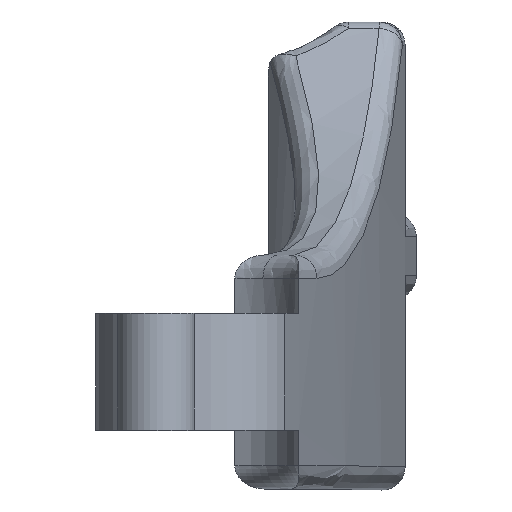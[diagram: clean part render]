
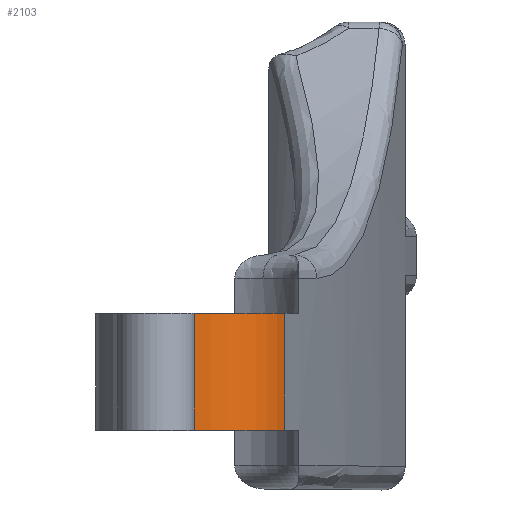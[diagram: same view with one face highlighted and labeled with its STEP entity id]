
A CAD part, top view. The second image highlights one B-rep face of the part: STEP entity #2103.
In plain terms, the highlighted cylindrical face has radius 12.6 mm (diameter 25.2 mm), a partial arc.
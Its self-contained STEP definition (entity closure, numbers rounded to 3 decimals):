
#48 = LINE ( 'NONE', #2157, #1083 ) ;
#54 = EDGE_LOOP ( 'NONE', ( #624, #430, #1079, #2313 ) ) ;
#61 = DIRECTION ( 'NONE',  ( 0., -1., 0. ) ) ;
#77 = DIRECTION ( 'NONE',  ( 0., 0., -1. ) ) ;
#184 = CARTESIAN_POINT ( 'NONE',  ( 0., 7.5, 110. ) ) ;
#252 = VERTEX_POINT ( 'NONE', #868 ) ;
#430 = ORIENTED_EDGE ( 'NONE', *, *, #2068, .T. ) ;
#481 = VERTEX_POINT ( 'NONE', #1852 ) ;
#607 = EDGE_CURVE ( 'NONE', #2057, #481, #1651, .T. ) ;
#624 = ORIENTED_EDGE ( 'NONE', *, *, #607, .T. ) ;
#700 = CARTESIAN_POINT ( 'NONE',  ( 0., 22.5, 110. ) ) ;
#797 = EDGE_CURVE ( 'NONE', #1496, #252, #1584, .T. ) ;
#868 = CARTESIAN_POINT ( 'NONE',  ( 0.037, 7.5, 122.6 ) ) ;
#874 = AXIS2_PLACEMENT_3D ( 'NONE', #700, #1478, #2463 ) ;
#1079 = ORIENTED_EDGE ( 'NONE', *, *, #797, .F. ) ;
#1083 = VECTOR ( 'NONE', #1208, 1000. ) ;
#1156 = CARTESIAN_POINT ( 'NONE',  ( 11.668, 7.5, 114.755 ) ) ;
#1175 = EDGE_CURVE ( 'NONE', #2057, #1496, #1524, .T. ) ;
#1184 = DIRECTION ( 'NONE',  ( 0., 0., -1. ) ) ;
#1208 = DIRECTION ( 'NONE',  ( 0., -1., 0. ) ) ;
#1381 = DIRECTION ( 'NONE',  ( 0., -1., 0. ) ) ;
#1478 = DIRECTION ( 'NONE',  ( 0., -1., 0. ) ) ;
#1496 = VERTEX_POINT ( 'NONE', #1156 ) ;
#1524 = LINE ( 'NONE', #1729, #2392 ) ;
#1584 = CIRCLE ( 'NONE', #1909, 12.6 ) ;
#1607 = CYLINDRICAL_SURFACE ( 'NONE', #2506, 12.6 ) ;
#1633 = CARTESIAN_POINT ( 'NONE',  ( 0., 60., 110. ) ) ;
#1646 = FACE_OUTER_BOUND ( 'NONE', #54, .T. ) ;
#1651 = CIRCLE ( 'NONE', #874, 12.6 ) ;
#1729 = CARTESIAN_POINT ( 'NONE',  ( 11.668, 60., 114.755 ) ) ;
#1806 = CARTESIAN_POINT ( 'NONE',  ( 11.668, 22.5, 114.755 ) ) ;
#1852 = CARTESIAN_POINT ( 'NONE',  ( 0.037, 22.5, 122.6 ) ) ;
#1909 = AXIS2_PLACEMENT_3D ( 'NONE', #184, #1381, #1184 ) ;
#2057 = VERTEX_POINT ( 'NONE', #1806 ) ;
#2068 = EDGE_CURVE ( 'NONE', #481, #252, #48, .T. ) ;
#2103 = ADVANCED_FACE ( 'NONE', ( #1646 ), #1607, .T. ) ;
#2157 = CARTESIAN_POINT ( 'NONE',  ( 0.037, 15., 122.6 ) ) ;
#2313 = ORIENTED_EDGE ( 'NONE', *, *, #1175, .F. ) ;
#2392 = VECTOR ( 'NONE', #2511, 1000. ) ;
#2463 = DIRECTION ( 'NONE',  ( 0., 0., -1. ) ) ;
#2506 = AXIS2_PLACEMENT_3D ( 'NONE', #1633, #61, #77 ) ;
#2511 = DIRECTION ( 'NONE',  ( 0., -1., 0. ) ) ;
